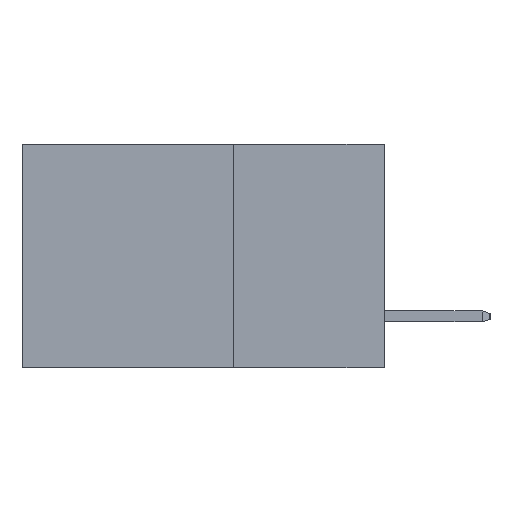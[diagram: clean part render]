
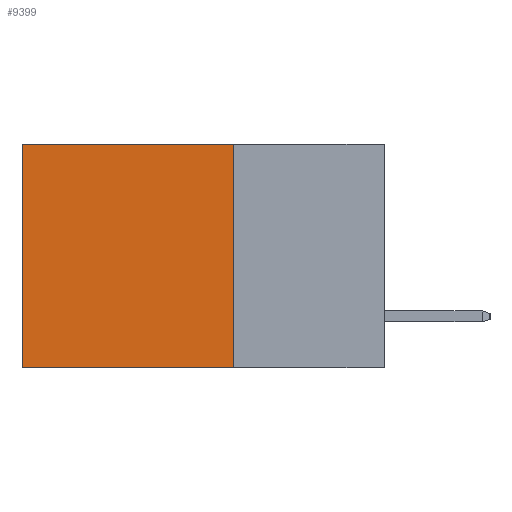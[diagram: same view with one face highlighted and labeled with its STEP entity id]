
A CAD part, left-side view. The second image highlights one B-rep face of the part: STEP entity #9399.
In plain terms, the highlighted planar face has unit normal (-1, 0, 0).
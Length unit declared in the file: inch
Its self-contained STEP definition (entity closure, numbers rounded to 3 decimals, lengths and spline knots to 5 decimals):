
#288 = ORIENTED_EDGE ( 'NONE', *, *, #15246, .F. ) ;
#296 = VECTOR ( 'NONE', #4219, 39.37008 ) ;
#534 = DIRECTION ( 'NONE',  ( 0., 0., -1. ) ) ;
#1124 = VECTOR ( 'NONE', #3323, 39.37008 ) ;
#1559 = AXIS2_PLACEMENT_3D ( 'NONE', #6896, #8156, #534 ) ;
#1726 = CARTESIAN_POINT ( 'NONE',  ( 0.298, 0.25, 0. ) ) ;
#1935 = LINE ( 'NONE', #9693, #1124 ) ;
#2796 = EDGE_CURVE ( 'NONE', #11504, #5124, #10386, .T. ) ;
#2920 = CARTESIAN_POINT ( 'NONE',  ( 0.298, 0.6, 0. ) ) ;
#3323 = DIRECTION ( 'NONE',  ( 0., 0., -1. ) ) ;
#4219 = DIRECTION ( 'NONE',  ( 0., 0., -1. ) ) ;
#5124 = VERTEX_POINT ( 'NONE', #9961 ) ;
#6043 = LINE ( 'NONE', #1726, #9445 ) ;
#6879 = DIRECTION ( 'NONE',  ( 0., 1., 0. ) ) ;
#6896 = CARTESIAN_POINT ( 'NONE',  ( 0.298, 0.25, 0. ) ) ;
#7078 = LINE ( 'NONE', #2920, #296 ) ;
#7214 = CARTESIAN_POINT ( 'NONE',  ( 0.298, 0.6, 0. ) ) ;
#7922 = ORIENTED_EDGE ( 'NONE', *, *, #2796, .F. ) ;
#8156 = DIRECTION ( 'NONE',  ( 1., 0., 0. ) ) ;
#8374 = CARTESIAN_POINT ( 'NONE',  ( 0.298, 0.25, 0. ) ) ;
#9017 = VERTEX_POINT ( 'NONE', #7214 ) ;
#9350 = EDGE_CURVE ( 'NONE', #9017, #5124, #7078, .T. ) ;
#9399 = ADVANCED_FACE ( 'NONE', ( #13058 ), #14526, .F. ) ;
#9445 = VECTOR ( 'NONE', #6879, 39.37008 ) ;
#9693 = CARTESIAN_POINT ( 'NONE',  ( 0.298, 0.25, 0. ) ) ;
#9961 = CARTESIAN_POINT ( 'NONE',  ( 0.298, 0.6, -0.37 ) ) ;
#10090 = EDGE_CURVE ( 'NONE', #13572, #9017, #6043, .T. ) ;
#10168 = DIRECTION ( 'NONE',  ( 0., 1., 0. ) ) ;
#10187 = CARTESIAN_POINT ( 'NONE',  ( 0.298, 0.25, -0.37 ) ) ;
#10198 = ORIENTED_EDGE ( 'NONE', *, *, #9350, .T. ) ;
#10386 = LINE ( 'NONE', #10187, #11214 ) ;
#11214 = VECTOR ( 'NONE', #10168, 39.37008 ) ;
#11504 = VERTEX_POINT ( 'NONE', #16293 ) ;
#13058 = FACE_OUTER_BOUND ( 'NONE', #13424, .T. ) ;
#13424 = EDGE_LOOP ( 'NONE', ( #10198, #7922, #288, #15993 ) ) ;
#13572 = VERTEX_POINT ( 'NONE', #8374 ) ;
#14526 = PLANE ( 'NONE',  #1559 ) ;
#15246 = EDGE_CURVE ( 'NONE', #13572, #11504, #1935, .T. ) ;
#15993 = ORIENTED_EDGE ( 'NONE', *, *, #10090, .T. ) ;
#16293 = CARTESIAN_POINT ( 'NONE',  ( 0.298, 0.25, -0.37 ) ) ;
